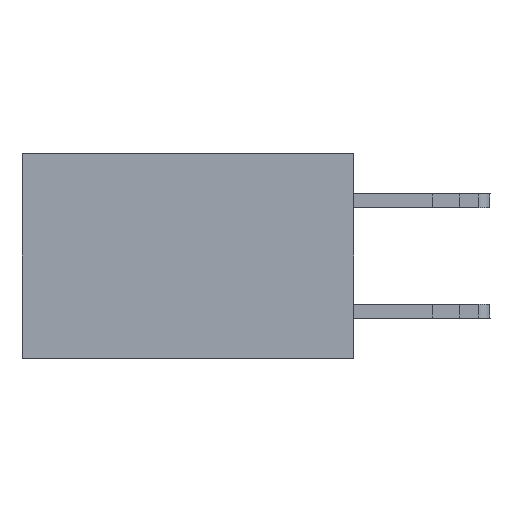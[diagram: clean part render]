
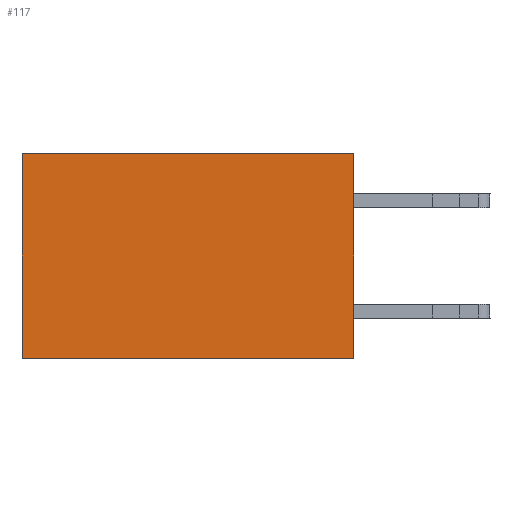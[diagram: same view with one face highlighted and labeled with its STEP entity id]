
A CAD part, left-side view. The second image highlights one B-rep face of the part: STEP entity #117.
In plain terms, the highlighted planar face has unit normal (-1, 0, 0).
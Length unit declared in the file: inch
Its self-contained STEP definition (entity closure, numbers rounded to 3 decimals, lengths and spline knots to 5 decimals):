
#117 = ADVANCED_FACE ( 'NONE', ( #1743 ), #11678, .F. ) ;
#331 = CARTESIAN_POINT ( 'NONE',  ( 0.2875, 0., 0. ) ) ;
#1602 = DIRECTION ( 'NONE',  ( 0., 0., -1. ) ) ;
#1743 = FACE_OUTER_BOUND ( 'NONE', #6140, .T. ) ;
#1938 = LINE ( 'NONE', #14629, #11461 ) ;
#2024 = DIRECTION ( 'NONE',  ( 1., 0., 0. ) ) ;
#2463 = DIRECTION ( 'NONE',  ( 0., 1., 0. ) ) ;
#2839 = AXIS2_PLACEMENT_3D ( 'NONE', #10504, #2024, #13313 ) ;
#3849 = VECTOR ( 'NONE', #1602, 39.37008 ) ;
#5605 = CARTESIAN_POINT ( 'NONE',  ( 0.2875, 0., 0. ) ) ;
#6140 = EDGE_LOOP ( 'NONE', ( #10783, #12194, #8274, #12396 ) ) ;
#6750 = VERTEX_POINT ( 'NONE', #5605 ) ;
#7148 = CARTESIAN_POINT ( 'NONE',  ( 0.2875, 0., -0.37 ) ) ;
#8000 = EDGE_CURVE ( 'NONE', #15461, #9881, #11300, .T. ) ;
#8274 = ORIENTED_EDGE ( 'NONE', *, *, #16433, .F. ) ;
#8887 = CARTESIAN_POINT ( 'NONE',  ( 0.2875, 0.6, 0. ) ) ;
#8942 = LINE ( 'NONE', #331, #3849 ) ;
#9881 = VERTEX_POINT ( 'NONE', #13577 ) ;
#10504 = CARTESIAN_POINT ( 'NONE',  ( 0.2875, 0., 0. ) ) ;
#10729 = DIRECTION ( 'NONE',  ( 0., 0., -1. ) ) ;
#10783 = ORIENTED_EDGE ( 'NONE', *, *, #8000, .T. ) ;
#11300 = LINE ( 'NONE', #17597, #15081 ) ;
#11461 = VECTOR ( 'NONE', #17358, 39.37008 ) ;
#11678 = PLANE ( 'NONE',  #2839 ) ;
#12194 = ORIENTED_EDGE ( 'NONE', *, *, #13328, .F. ) ;
#12396 = ORIENTED_EDGE ( 'NONE', *, *, #14573, .T. ) ;
#13313 = DIRECTION ( 'NONE',  ( 0., 0., -1. ) ) ;
#13328 = EDGE_CURVE ( 'NONE', #17519, #9881, #17727, .T. ) ;
#13577 = CARTESIAN_POINT ( 'NONE',  ( 0.2875, 0.6, -0.37 ) ) ;
#14573 = EDGE_CURVE ( 'NONE', #6750, #15461, #1938, .T. ) ;
#14616 = CARTESIAN_POINT ( 'NONE',  ( 0.2875, 0., -0.37 ) ) ;
#14629 = CARTESIAN_POINT ( 'NONE',  ( 0.2875, 0., 0. ) ) ;
#15081 = VECTOR ( 'NONE', #10729, 39.37008 ) ;
#15461 = VERTEX_POINT ( 'NONE', #8887 ) ;
#16433 = EDGE_CURVE ( 'NONE', #6750, #17519, #8942, .T. ) ;
#17277 = VECTOR ( 'NONE', #2463, 39.37008 ) ;
#17358 = DIRECTION ( 'NONE',  ( 0., 1., 0. ) ) ;
#17519 = VERTEX_POINT ( 'NONE', #7148 ) ;
#17597 = CARTESIAN_POINT ( 'NONE',  ( 0.2875, 0.6, 0. ) ) ;
#17727 = LINE ( 'NONE', #14616, #17277 ) ;
